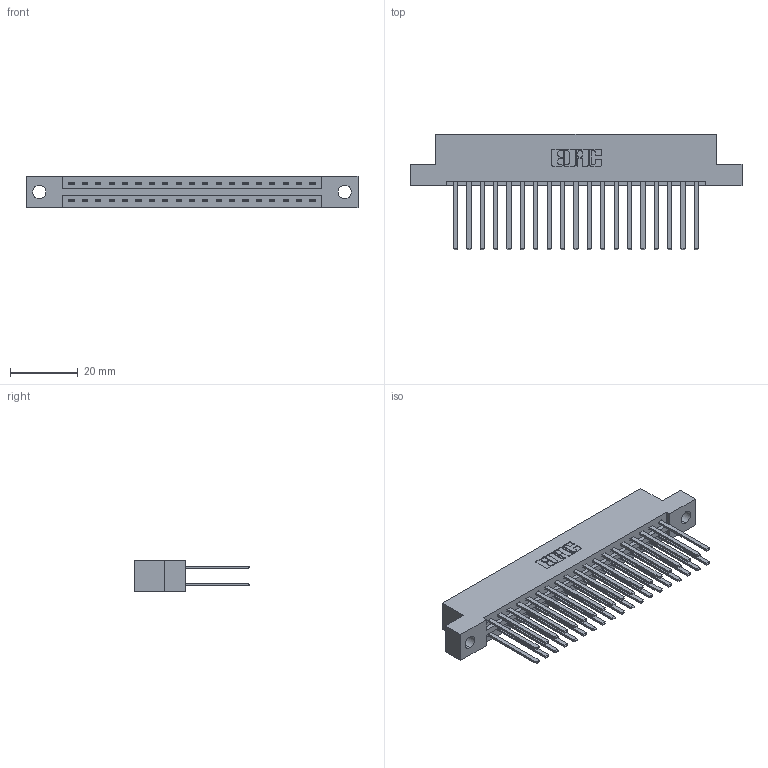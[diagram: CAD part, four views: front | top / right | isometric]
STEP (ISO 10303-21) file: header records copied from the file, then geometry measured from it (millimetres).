
FILE_DESCRIPTION (( 'STEP AP203' ), '1' );
FILE_NAME ('387-038-544-204.STEP', '2019-10-17T21:50:38', ( '' ), ( '' ), 'SwSTEP 2.0', 'SolidWorks 2016', '' );
FILE_SCHEMA (( 'CONFIG_CONTROL_DESIGN' ));
Length unit declared in the file: inch
Products named in the file (3): 387-038-544-204; 337 Part_Flush Mounting Lugs - 0.156 Dia-TH; 345-292-001_345-293-144
Assembly tree (39 placements, depth 2):
  387-038-544-204
    337 Part_Flush Mounting Lugs - 0.156 Dia-TH
    345-292-001_345-293-144  x38
Bounding box: 98.3 x 34.3 x 9.4 mm (x, y, z)
Volume: 10498.1 mm3; surface area: 13182.3 mm2
Topology: 39 solids, 39 shells, 1938 faces, 5745 edges, 3778 vertices
Faces by surface type: plane 1362, cylinder 576
Entity records: 17525 total; most frequent: CARTESIAN_POINT 2970, ORIENTED_EDGE 2906, DIRECTION 2565, EDGE_CURVE 1453, LINE 1329, VECTOR 1329, VERTEX_POINT 966, AXIS2_PLACEMENT_3D 618
